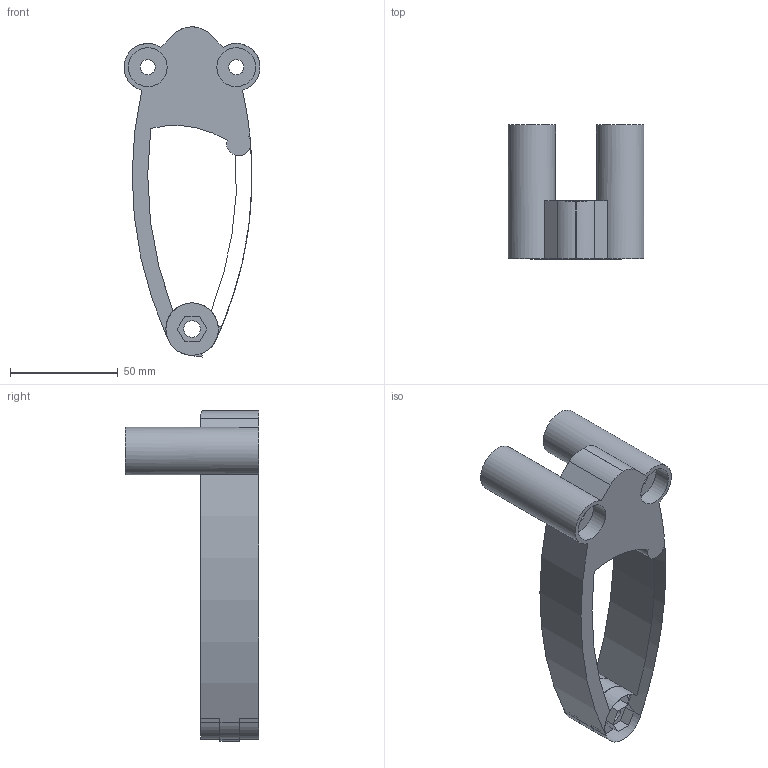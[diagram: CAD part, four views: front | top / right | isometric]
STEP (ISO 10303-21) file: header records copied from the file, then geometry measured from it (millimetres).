
FILE_DESCRIPTION(('FreeCAD Model'),'2;1');
FILE_NAME('('Author'),(''), 'Open CASCADE STEP processor 6.8','FreeCAD','Unknown');
FILE_SCHEMA(('AUTOMOTIVE_DESIGN_CC2 { 1 2 10303 214 -1 1 5 4 }'));
Length unit declared in the file: millimetre
Products named in the file (2): Pocket010; Pocket009
Bounding box: 63 x 62.01 x 153.08 mm (x, y, z)
Volume: 124833.2 mm3; surface area: 36802.6 mm2
Topology: 2 solids, 2 shells, 85 faces, 214 edges, 138 vertices
Faces by surface type: cylinder 47, plane 38
Full cylindrical faces by diameter (mm): 7 x2, 15 x2, 18 x2, 22 x2
Entity records: 8771 total; most frequent: CARTESIAN_POINT 4722, DIRECTION 689, ORIENTED_EDGE 428, PCURVE 428, DEFINITIONAL_REPRESENTATION 428, LINE 245, VECTOR 245, EDGE_CURVE 214
